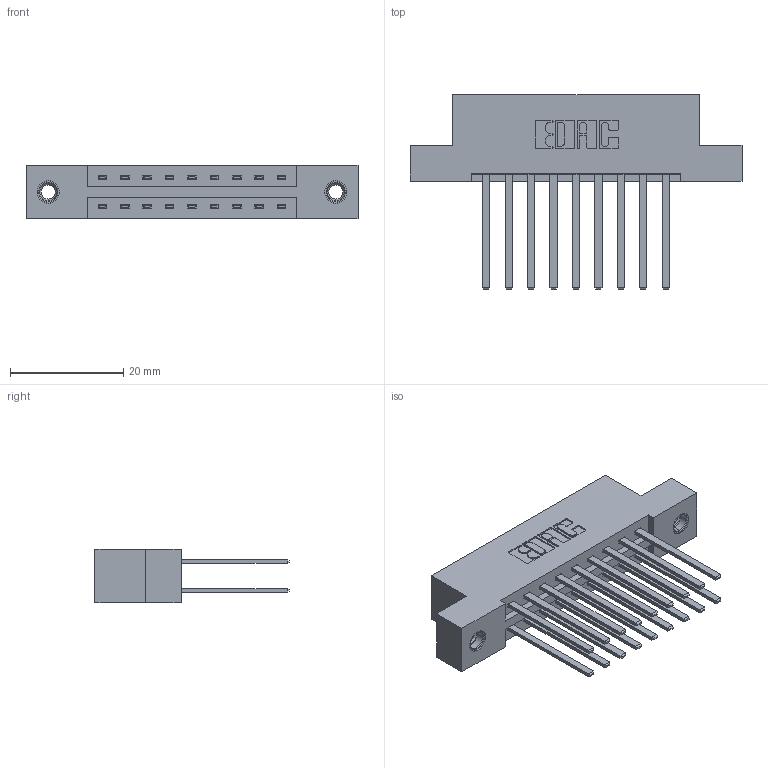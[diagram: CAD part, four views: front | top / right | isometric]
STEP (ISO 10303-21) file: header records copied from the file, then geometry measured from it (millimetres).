
FILE_DESCRIPTION (( 'STEP AP203' ), '1' );
FILE_NAME ('337-018-544-207.STEP', '2019-10-08T13:20:07', ( '' ), ( '' ), 'SwSTEP 2.0', 'SolidWorks 2016', '' );
FILE_SCHEMA (( 'CONFIG_CONTROL_DESIGN' ));
Length unit declared in the file: inch
Products named in the file (4): 337 Part_Flush Mounting Lugs - 0.156 Dia-TI; 345-292-001_345-293-144; 345-250-001_345-250-005-103; 337-018-544-207
Assembly tree (21 placements, depth 2):
  337-018-544-207
    337 Part_Flush Mounting Lugs - 0.156 Dia-TI
    345-292-001_345-293-144  x18
    345-250-001_345-250-005-103  x2
Bounding box: 58.67 x 34.3 x 9.4 mm (x, y, z)
Volume: 5983.1 mm3; surface area: 7303.6 mm2
Topology: 21 solids, 21 shells, 1038 faces, 3021 edges, 1982 vertices
Faces by surface type: plane 714, cylinder 308, cone 12, torus 4
Entity records: 12248 total; most frequent: CARTESIAN_POINT 2069, ORIENTED_EDGE 1998, DIRECTION 1849, EDGE_CURVE 999, VECTOR 855, LINE 855, VERTEX_POINT 660, AXIS2_PLACEMENT_3D 497
